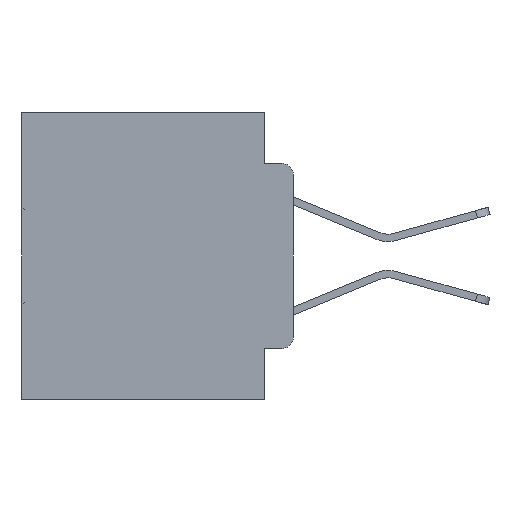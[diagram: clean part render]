
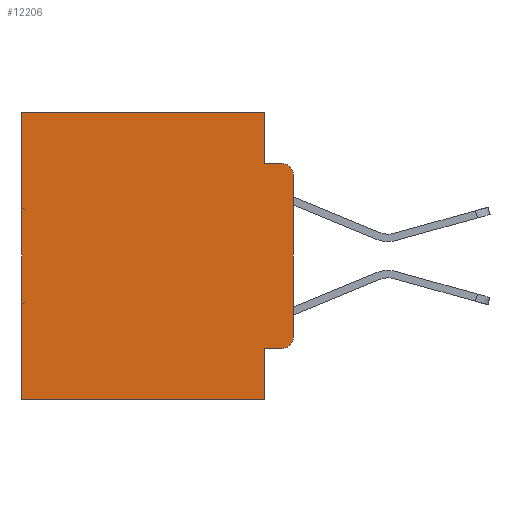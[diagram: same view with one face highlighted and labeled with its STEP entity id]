
A CAD part, left-side view. The second image highlights one B-rep face of the part: STEP entity #12206.
In plain terms, the highlighted planar face has unit normal (-1, 0, 0).
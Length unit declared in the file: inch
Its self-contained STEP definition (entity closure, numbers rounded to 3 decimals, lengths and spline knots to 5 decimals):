
#442 = DIRECTION ( 'NONE',  ( 0., -1., 0. ) ) ;
#791 = ORIENTED_EDGE ( 'NONE', *, *, #22550, .T. ) ;
#1262 = CARTESIAN_POINT ( 'NONE',  ( 0.298, 0.473, 0. ) ) ;
#1398 = CARTESIAN_POINT ( 'NONE',  ( 0.298, 0.051, -0.4115 ) ) ;
#2115 = CARTESIAN_POINT ( 'NONE',  ( 0.298, 0.051, 0. ) ) ;
#2349 = VERTEX_POINT ( 'NONE', #19221 ) ;
#2686 = DIRECTION ( 'NONE',  ( 0., 1., 0. ) ) ;
#2867 = ORIENTED_EDGE ( 'NONE', *, *, #27953, .T. ) ;
#3285 = VECTOR ( 'NONE', #13633, 39.37008 ) ;
#3753 = DIRECTION ( 'NONE',  ( -1., 0., 0. ) ) ;
#4148 = LINE ( 'NONE', #24017, #3285 ) ;
#4446 = PLANE ( 'NONE',  #27121 ) ;
#6360 = EDGE_CURVE ( 'NONE', #23487, #15293, #14844, .T. ) ;
#6663 = ORIENTED_EDGE ( 'NONE', *, *, #19638, .F. ) ;
#7490 = EDGE_CURVE ( 'NONE', #29550, #23768, #30030, .T. ) ;
#7912 = CARTESIAN_POINT ( 'NONE',  ( 0.298, 0., -0.3915 ) ) ;
#8622 = CARTESIAN_POINT ( 'NONE',  ( 0.298, 0.02, -0.4115 ) ) ;
#9357 = VECTOR ( 'NONE', #24793, 39.37008 ) ;
#9754 = DIRECTION ( 'NONE',  ( 0., 0., -1. ) ) ;
#9897 = ORIENTED_EDGE ( 'NONE', *, *, #23889, .F. ) ;
#9995 = DIRECTION ( 'NONE',  ( 0., 0., -1. ) ) ;
#11100 = CARTESIAN_POINT ( 'NONE',  ( 0.298, 0.051, -0.0885 ) ) ;
#11125 = VECTOR ( 'NONE', #23669, 39.37008 ) ;
#11732 = DIRECTION ( 'NONE',  ( 0., -1., 0. ) ) ;
#12206 = ADVANCED_FACE ( 'NONE', ( #13762 ), #4446, .F. ) ;
#12376 = CARTESIAN_POINT ( 'NONE',  ( 0.298, 0.473, 0. ) ) ;
#12681 = LINE ( 'NONE', #11100, #32449 ) ;
#13223 = CARTESIAN_POINT ( 'NONE',  ( 0.298, 0., -0.5 ) ) ;
#13480 = LINE ( 'NONE', #13223, #18887 ) ;
#13619 = VECTOR ( 'NONE', #15963, 39.37008 ) ;
#13633 = DIRECTION ( 'NONE',  ( 0., 0., -1. ) ) ;
#13721 = DIRECTION ( 'NONE',  ( -1., 0., 0. ) ) ;
#13762 = FACE_OUTER_BOUND ( 'NONE', #33389, .T. ) ;
#14441 = ORIENTED_EDGE ( 'NONE', *, *, #7490, .F. ) ;
#14844 = LINE ( 'NONE', #2115, #33692 ) ;
#15210 = EDGE_CURVE ( 'NONE', #29673, #25727, #18221, .T. ) ;
#15293 = VERTEX_POINT ( 'NONE', #28988 ) ;
#15963 = DIRECTION ( 'NONE',  ( 0., 1., 0. ) ) ;
#18221 = LINE ( 'NONE', #12376, #11125 ) ;
#18887 = VECTOR ( 'NONE', #2686, 39.37008 ) ;
#19221 = CARTESIAN_POINT ( 'NONE',  ( 0.298, 0.051, -0.0885 ) ) ;
#19378 = AXIS2_PLACEMENT_3D ( 'NONE', #19591, #3753, #22160 ) ;
#19414 = ORIENTED_EDGE ( 'NONE', *, *, #22180, .F. ) ;
#19591 = CARTESIAN_POINT ( 'NONE',  ( 0.298, 0.02, -0.1085 ) ) ;
#19599 = CARTESIAN_POINT ( 'NONE',  ( 0.298, 0.051, -0.4115 ) ) ;
#19638 = EDGE_CURVE ( 'NONE', #15293, #25727, #13480, .T. ) ;
#20618 = ORIENTED_EDGE ( 'NONE', *, *, #6360, .F. ) ;
#21431 = CIRCLE ( 'NONE', #19378, 0.02 ) ;
#21892 = CARTESIAN_POINT ( 'NONE',  ( 0.298, 0., -0.1085 ) ) ;
#22160 = DIRECTION ( 'NONE',  ( 0., 0., -1. ) ) ;
#22180 = EDGE_CURVE ( 'NONE', #23330, #2349, #4148, .T. ) ;
#22213 = CARTESIAN_POINT ( 'NONE',  ( 0.298, 0., 0. ) ) ;
#22248 = ORIENTED_EDGE ( 'NONE', *, *, #31329, .T. ) ;
#22550 = EDGE_CURVE ( 'NONE', #23330, #29673, #28215, .T. ) ;
#22806 = CARTESIAN_POINT ( 'NONE',  ( 0.298, 0., 0. ) ) ;
#23330 = VERTEX_POINT ( 'NONE', #31803 ) ;
#23487 = VERTEX_POINT ( 'NONE', #1398 ) ;
#23669 = DIRECTION ( 'NONE',  ( 0., 0., -1. ) ) ;
#23768 = VERTEX_POINT ( 'NONE', #7912 ) ;
#23889 = EDGE_CURVE ( 'NONE', #2349, #32416, #12681, .T. ) ;
#24017 = CARTESIAN_POINT ( 'NONE',  ( 0.298, 0.051, 0. ) ) ;
#24103 = VECTOR ( 'NONE', #11732, 39.37008 ) ;
#24793 = DIRECTION ( 'NONE',  ( 0., 0., -1. ) ) ;
#25392 = DIRECTION ( 'NONE',  ( 1., 0., 0. ) ) ;
#25727 = VERTEX_POINT ( 'NONE', #29904 ) ;
#25836 = ORIENTED_EDGE ( 'NONE', *, *, #15210, .T. ) ;
#27121 = AXIS2_PLACEMENT_3D ( 'NONE', #22806, #25392, #9754 ) ;
#27903 = CARTESIAN_POINT ( 'NONE',  ( 0.298, 0., 0. ) ) ;
#27953 = EDGE_CURVE ( 'NONE', #33626, #23768, #29450, .T. ) ;
#28202 = ORIENTED_EDGE ( 'NONE', *, *, #29002, .T. ) ;
#28215 = LINE ( 'NONE', #27903, #13619 ) ;
#28988 = CARTESIAN_POINT ( 'NONE',  ( 0.298, 0.051, -0.5 ) ) ;
#29002 = EDGE_CURVE ( 'NONE', #29550, #32416, #21431, .T. ) ;
#29210 = CARTESIAN_POINT ( 'NONE',  ( 0.298, 0.02, -0.3915 ) ) ;
#29450 = CIRCLE ( 'NONE', #32132, 0.02 ) ;
#29550 = VERTEX_POINT ( 'NONE', #21892 ) ;
#29673 = VERTEX_POINT ( 'NONE', #1262 ) ;
#29904 = CARTESIAN_POINT ( 'NONE',  ( 0.298, 0.473, -0.5 ) ) ;
#30030 = LINE ( 'NONE', #22213, #9357 ) ;
#30069 = LINE ( 'NONE', #19599, #24103 ) ;
#31329 = EDGE_CURVE ( 'NONE', #23487, #33626, #30069, .T. ) ;
#31641 = CARTESIAN_POINT ( 'NONE',  ( 0.298, 0.02, -0.0885 ) ) ;
#31738 = DIRECTION ( 'NONE',  ( 0., 0., -1. ) ) ;
#31803 = CARTESIAN_POINT ( 'NONE',  ( 0.298, 0.051, 0. ) ) ;
#32132 = AXIS2_PLACEMENT_3D ( 'NONE', #29210, #13721, #31738 ) ;
#32416 = VERTEX_POINT ( 'NONE', #31641 ) ;
#32449 = VECTOR ( 'NONE', #442, 39.37008 ) ;
#33389 = EDGE_LOOP ( 'NONE', ( #14441, #28202, #9897, #19414, #791, #25836, #6663, #20618, #22248, #2867 ) ) ;
#33626 = VERTEX_POINT ( 'NONE', #8622 ) ;
#33692 = VECTOR ( 'NONE', #9995, 39.37008 ) ;
